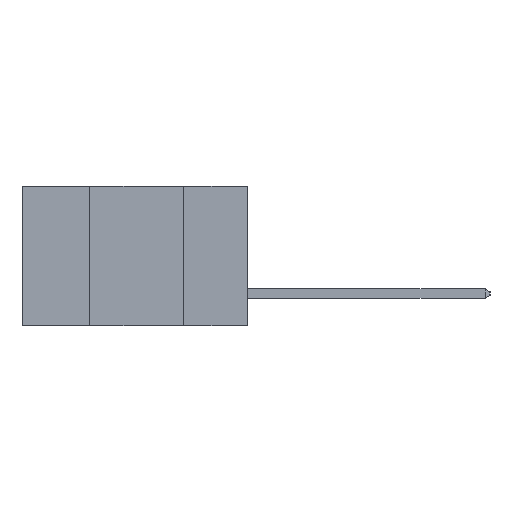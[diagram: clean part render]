
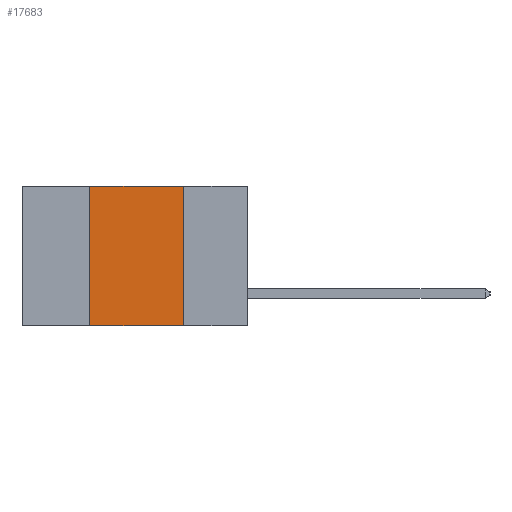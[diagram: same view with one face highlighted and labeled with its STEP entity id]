
A CAD part, left-side view. The second image highlights one B-rep face of the part: STEP entity #17683.
In plain terms, the highlighted planar face has unit normal (-1, 0, 0).
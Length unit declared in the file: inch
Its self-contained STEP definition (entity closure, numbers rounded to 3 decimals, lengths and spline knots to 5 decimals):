
#350 = DIRECTION ( 'NONE',  ( 0., 0., -1. ) ) ;
#839 = DIRECTION ( 'NONE',  ( 0., -1., 0. ) ) ;
#1472 = LINE ( 'NONE', #21580, #12063 ) ;
#1948 = CARTESIAN_POINT ( 'NONE',  ( 0., 0.42, 0. ) ) ;
#3220 = ORIENTED_EDGE ( 'NONE', *, *, #21881, .F. ) ;
#4009 = CARTESIAN_POINT ( 'NONE',  ( 0., 0.42, 0. ) ) ;
#4347 = LINE ( 'NONE', #13325, #9333 ) ;
#5275 = CARTESIAN_POINT ( 'NONE',  ( 0., 0.17, 0. ) ) ;
#6324 = EDGE_CURVE ( 'NONE', #7286, #24908, #1472, .T. ) ;
#6367 = ORIENTED_EDGE ( 'NONE', *, *, #6324, .F. ) ;
#7286 = VERTEX_POINT ( 'NONE', #1948 ) ;
#8788 = ORIENTED_EDGE ( 'NONE', *, *, #14155, .F. ) ;
#8856 = PLANE ( 'NONE',  #20878 ) ;
#9333 = VECTOR ( 'NONE', #23749, 39.37008 ) ;
#9563 = VECTOR ( 'NONE', #12390, 39.37008 ) ;
#10356 = VECTOR ( 'NONE', #22872, 39.37008 ) ;
#10874 = LINE ( 'NONE', #4009, #9563 ) ;
#10960 = CARTESIAN_POINT ( 'NONE',  ( 0., 0.6, 0. ) ) ;
#12063 = VECTOR ( 'NONE', #839, 39.37008 ) ;
#12390 = DIRECTION ( 'NONE',  ( 0., 0., 1. ) ) ;
#12522 = VERTEX_POINT ( 'NONE', #24293 ) ;
#13042 = DIRECTION ( 'NONE',  ( 1., 0., 0. ) ) ;
#13325 = CARTESIAN_POINT ( 'NONE',  ( 0., 0.17, 0. ) ) ;
#14155 = EDGE_CURVE ( 'NONE', #12522, #7286, #10874, .T. ) ;
#14397 = ORIENTED_EDGE ( 'NONE', *, *, #21640, .T. ) ;
#15425 = VERTEX_POINT ( 'NONE', #24647 ) ;
#17683 = ADVANCED_FACE ( 'NONE', ( #21110 ), #8856, .F. ) ;
#20878 = AXIS2_PLACEMENT_3D ( 'NONE', #10960, #13042, #350 ) ;
#21110 = FACE_OUTER_BOUND ( 'NONE', #25795, .T. ) ;
#21580 = CARTESIAN_POINT ( 'NONE',  ( 0., 0.6, 0. ) ) ;
#21640 = EDGE_CURVE ( 'NONE', #12522, #15425, #26822, .T. ) ;
#21881 = EDGE_CURVE ( 'NONE', #24908, #15425, #4347, .T. ) ;
#22872 = DIRECTION ( 'NONE',  ( 0., -1., 0. ) ) ;
#23749 = DIRECTION ( 'NONE',  ( 0., 0., -1. ) ) ;
#24293 = CARTESIAN_POINT ( 'NONE',  ( 0., 0.42, -0.37 ) ) ;
#24647 = CARTESIAN_POINT ( 'NONE',  ( 0., 0.17, -0.37 ) ) ;
#24908 = VERTEX_POINT ( 'NONE', #5275 ) ;
#25795 = EDGE_LOOP ( 'NONE', ( #3220, #6367, #8788, #14397 ) ) ;
#26822 = LINE ( 'NONE', #26975, #10356 ) ;
#26975 = CARTESIAN_POINT ( 'NONE',  ( 0., 0.6, -0.37 ) ) ;
